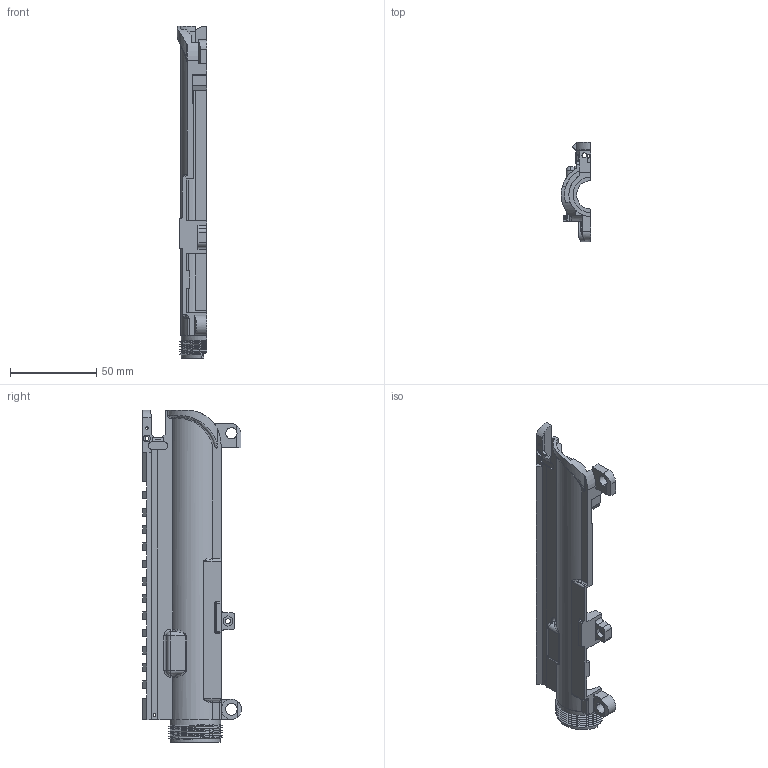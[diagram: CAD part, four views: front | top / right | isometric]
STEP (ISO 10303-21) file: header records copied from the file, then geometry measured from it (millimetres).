
FILE_DESCRIPTION (( 'STEP AP203' ), '1' );
FILE_NAME ('xr15_upper_l.STEP', '2021-12-29T04:23:35', ( '' ), ( '' ), 'SwSTEP 2.0', 'SolidWorks 2015', '' );
FILE_SCHEMA (( 'CONFIG_CONTROL_DESIGN' ));
Length unit declared in the file: millimetre
Products named in the file (1): xr15_upper_l
Bounding box: 17.24 x 57.3 x 192.5 mm (x, y, z)
Volume: 31972.9 mm3; surface area: 26572.2 mm2
Topology: 1 solids, 1 shells, 310 faces, 852 edges, 539 vertices
Faces by surface type: plane 185, cylinder 88, bspline 21, torus 11, sphere 4, cone 1
Entity records: 13117 total; most frequent: CARTESIAN_POINT 5305, ORIENTED_EDGE 1696, DIRECTION 1522, EDGE_CURVE 848, LINE 572, VECTOR 572, VERTEX_POINT 539, AXIS2_PLACEMENT_3D 475
